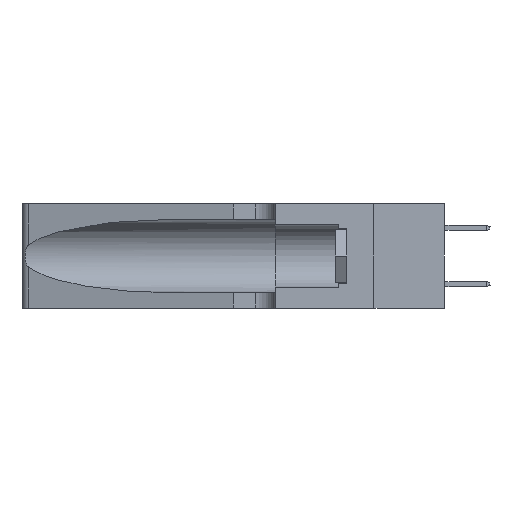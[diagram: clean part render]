
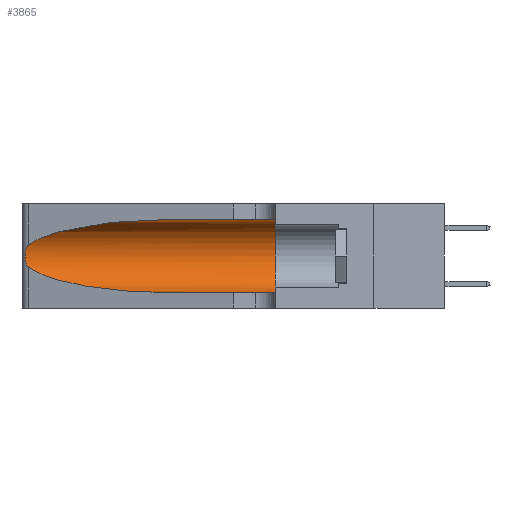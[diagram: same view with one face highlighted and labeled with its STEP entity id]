
A CAD part, left-side view. The second image highlights one B-rep face of the part: STEP entity #3865.
In plain terms, the highlighted cylindrical face has radius 3.308 mm (diameter 6.617 mm), a partial arc.
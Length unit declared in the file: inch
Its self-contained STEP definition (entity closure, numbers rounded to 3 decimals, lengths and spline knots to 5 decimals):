
#106 = DIRECTION ( 'NONE',  ( 0., -1., 0. ) ) ;
#166 = CARTESIAN_POINT ( 'NONE',  ( 0.25487, 1.22718, 0.22369 ) ) ;
#390 = CIRCLE ( 'NONE', #15256, 0.13025 ) ;
#1491 = CARTESIAN_POINT ( 'NONE',  ( 0.25856, 1.23593, 0.16098 ) ) ;
#1495 = CARTESIAN_POINT ( 'NONE',  ( 0.1305, 0.72297, 0.31525 ) ) ;
#1631 = CARTESIAN_POINT ( 'NONE',  ( 0.18966, 0.96281, 0.05475 ) ) ;
#2204 = ORIENTED_EDGE ( 'NONE', *, *, #9505, .F. ) ;
#2367 = CYLINDRICAL_SURFACE ( 'NONE', #14050, 0.13025 ) ;
#2941 = ORIENTED_EDGE ( 'NONE', *, *, #15355, .T. ) ;
#2947 = B_SPLINE_CURVE_WITH_KNOTS ( 'NONE', 3,
 ( #18008, #19678, #6514, #18069, #8222, #19756, #9849, #21394, #11514, #1491, #13173, #3213, #14814, #4909 ),
 .UNSPECIFIED., .F., .F.,
 ( 4, 2, 2, 2, 2, 2, 4 ),
 ( 0., 0.00027, 0.00053, 0.00107, 0.0016, 0.00187, 0.00214 ),
 .UNSPECIFIED. ) ;
#3213 = CARTESIAN_POINT ( 'NONE',  ( 0.25639, 1.23186, 0.15144 ) ) ;
#3232 =( BOUNDED_CURVE ( )  B_SPLINE_CURVE ( 3, ( #20146, #8592, #10243, #166 ),
 .UNSPECIFIED., .F., .F. ) 
 B_SPLINE_CURVE_WITH_KNOTS ( ( 4, 4 ),
 ( 1.5708, 2.84003 ),
 .UNSPECIFIED. ) 
 CURVE ( )  GEOMETRIC_REPRESENTATION_ITEM ( )  RATIONAL_B_SPLINE_CURVE ( ( 1., 0.87, 0.87, 1. ) ) 
 REPRESENTATION_ITEM ( '' )  );
#3292 = CARTESIAN_POINT ( 'NONE',  ( 0.2373, 1.15595, 0.08982 ) ) ;
#3432 = VERTEX_POINT ( 'NONE', #10956 ) ;
#3658 = DIRECTION ( 'NONE',  ( 0., 0., -1. ) ) ;
#3820 = DIRECTION ( 'NONE',  ( 0., -1., 0. ) ) ;
#3865 = ADVANCED_FACE ( 'NONE', ( #15628 ), #2367, .F. ) ;
#4185 =( BOUNDED_CURVE ( )  B_SPLINE_CURVE ( 3, ( #21531, #3292, #1631, #13312 ),
 .UNSPECIFIED., .F., .T. ) 
 B_SPLINE_CURVE_WITH_KNOTS ( ( 4, 4 ),
 ( 3.44316, 4.71239 ),
 .UNSPECIFIED. ) 
 CURVE ( )  GEOMETRIC_REPRESENTATION_ITEM ( )  RATIONAL_B_SPLINE_CURVE ( ( 1., 0.87, 0.87, 1. ) ) 
 REPRESENTATION_ITEM ( '' )  );
#4385 = CARTESIAN_POINT ( 'NONE',  ( 0.1305, 0.35, 0.05475 ) ) ;
#4403 = VECTOR ( 'NONE', #106, 39.37008 ) ;
#4891 = VERTEX_POINT ( 'NONE', #10498 ) ;
#4909 = CARTESIAN_POINT ( 'NONE',  ( 0.25487, 1.22718, 0.14631 ) ) ;
#6455 = CARTESIAN_POINT ( 'NONE',  ( 0.1305, 0.35, 0.185 ) ) ;
#6514 = CARTESIAN_POINT ( 'NONE',  ( 0.25639, 1.23184, 0.21858 ) ) ;
#6599 = EDGE_CURVE ( 'NONE', #3432, #14009, #4185, .T. ) ;
#6842 = CARTESIAN_POINT ( 'NONE',  ( 0.1305, 1.61858, 0.31525 ) ) ;
#8163 = DIRECTION ( 'NONE',  ( 0., 0., 1. ) ) ;
#8222 = CARTESIAN_POINT ( 'NONE',  ( 0.25854, 1.2359, 0.20912 ) ) ;
#8592 = CARTESIAN_POINT ( 'NONE',  ( 0.18966, 0.96281, 0.31525 ) ) ;
#8636 = DIRECTION ( 'NONE',  ( 0., -1., 0. ) ) ;
#8845 = LINE ( 'NONE', #6842, #4403 ) ;
#9505 = EDGE_CURVE ( 'NONE', #4891, #11972, #390, .T. ) ;
#9607 = ORIENTED_EDGE ( 'NONE', *, *, #20392, .F. ) ;
#9849 = CARTESIAN_POINT ( 'NONE',  ( 0.26075, 1.23896, 0.19203 ) ) ;
#9903 = ORIENTED_EDGE ( 'NONE', *, *, #11487, .T. ) ;
#10243 = CARTESIAN_POINT ( 'NONE',  ( 0.2373, 1.15595, 0.28018 ) ) ;
#10498 = CARTESIAN_POINT ( 'NONE',  ( 0.1305, 0.35, 0.31525 ) ) ;
#10819 = ORIENTED_EDGE ( 'NONE', *, *, #6599, .T. ) ;
#10956 = CARTESIAN_POINT ( 'NONE',  ( 0.25487, 1.22718, 0.14631 ) ) ;
#11021 = EDGE_CURVE ( 'NONE', #15699, #14003, #3232, .T. ) ;
#11487 = EDGE_CURVE ( 'NONE', #14003, #3432, #2947, .T. ) ;
#11514 = CARTESIAN_POINT ( 'NONE',  ( 0.26017, 1.23833, 0.17102 ) ) ;
#11972 = VERTEX_POINT ( 'NONE', #4385 ) ;
#13136 = EDGE_LOOP ( 'NONE', ( #13327, #9903, #10819, #2941, #2204, #9607 ) ) ;
#13173 = CARTESIAN_POINT ( 'NONE',  ( 0.25789, 1.23486, 0.15765 ) ) ;
#13312 = CARTESIAN_POINT ( 'NONE',  ( 0.1305, 0.72297, 0.05475 ) ) ;
#13327 = ORIENTED_EDGE ( 'NONE', *, *, #11021, .T. ) ;
#14003 = VERTEX_POINT ( 'NONE', #18643 ) ;
#14009 = VERTEX_POINT ( 'NONE', #17041 ) ;
#14050 = AXIS2_PLACEMENT_3D ( 'NONE', #15243, #8636, #3658 ) ;
#14814 = CARTESIAN_POINT ( 'NONE',  ( 0.25555, 1.22993, 0.14849 ) ) ;
#15243 = CARTESIAN_POINT ( 'NONE',  ( 0.1305, 1.61858, 0.185 ) ) ;
#15256 = AXIS2_PLACEMENT_3D ( 'NONE', #6455, #18015, #8163 ) ;
#15355 = EDGE_CURVE ( 'NONE', #14009, #11972, #20643, .T. ) ;
#15628 = FACE_OUTER_BOUND ( 'NONE', #13136, .T. ) ;
#15699 = VERTEX_POINT ( 'NONE', #1495 ) ;
#16228 = VECTOR ( 'NONE', #3820, 39.37008 ) ;
#17041 = CARTESIAN_POINT ( 'NONE',  ( 0.1305, 0.72297, 0.05475 ) ) ;
#18008 = CARTESIAN_POINT ( 'NONE',  ( 0.25487, 1.22718, 0.22369 ) ) ;
#18015 = DIRECTION ( 'NONE',  ( 0., 1., 0. ) ) ;
#18069 = CARTESIAN_POINT ( 'NONE',  ( 0.25787, 1.23484, 0.2124 ) ) ;
#18643 = CARTESIAN_POINT ( 'NONE',  ( 0.25487, 1.22718, 0.22369 ) ) ;
#18665 = CARTESIAN_POINT ( 'NONE',  ( 0.1305, 1.61858, 0.05475 ) ) ;
#19678 = CARTESIAN_POINT ( 'NONE',  ( 0.25555, 1.22994, 0.2215 ) ) ;
#19756 = CARTESIAN_POINT ( 'NONE',  ( 0.26018, 1.23835, 0.19895 ) ) ;
#20146 = CARTESIAN_POINT ( 'NONE',  ( 0.1305, 0.72297, 0.31525 ) ) ;
#20392 = EDGE_CURVE ( 'NONE', #15699, #4891, #8845, .T. ) ;
#20643 = LINE ( 'NONE', #18665, #16228 ) ;
#21394 = CARTESIAN_POINT ( 'NONE',  ( 0.26075, 1.23896, 0.178 ) ) ;
#21531 = CARTESIAN_POINT ( 'NONE',  ( 0.25487, 1.22718, 0.14631 ) ) ;
